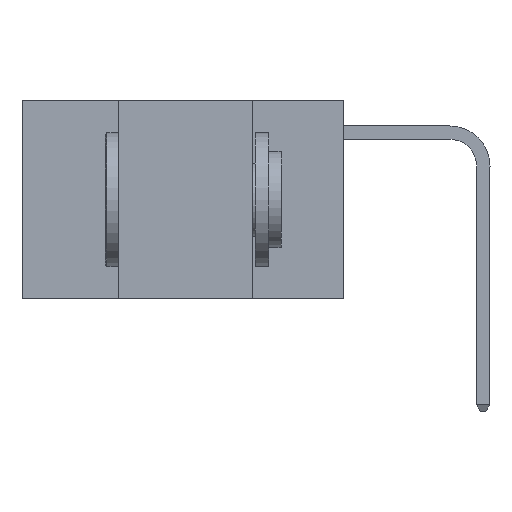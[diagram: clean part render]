
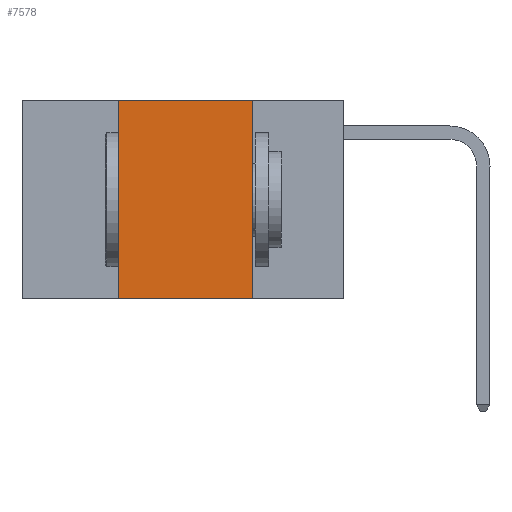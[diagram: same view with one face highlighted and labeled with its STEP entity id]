
A CAD part, left-side view. The second image highlights one B-rep face of the part: STEP entity #7578.
In plain terms, the highlighted planar face has unit normal (-1, 0, 0).
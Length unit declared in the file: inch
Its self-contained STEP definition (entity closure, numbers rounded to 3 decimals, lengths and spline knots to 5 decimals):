
#223 = DIRECTION ( 'NONE',  ( 0., -1., 0. ) ) ;
#427 = CARTESIAN_POINT ( 'NONE',  ( 0., 0.42, 0. ) ) ;
#660 = ORIENTED_EDGE ( 'NONE', *, *, #11744, .T. ) ;
#1587 = CARTESIAN_POINT ( 'NONE',  ( 0., 0.6, -0.37 ) ) ;
#1807 = DIRECTION ( 'NONE',  ( 1., 0., 0. ) ) ;
#2647 = CARTESIAN_POINT ( 'NONE',  ( 0., 0.17, 0. ) ) ;
#3037 = VERTEX_POINT ( 'NONE', #427 ) ;
#3234 = VERTEX_POINT ( 'NONE', #17712 ) ;
#4176 = CARTESIAN_POINT ( 'NONE',  ( 0., 0.17, 0. ) ) ;
#4895 = VECTOR ( 'NONE', #8640, 39.37008 ) ;
#5818 = CARTESIAN_POINT ( 'NONE',  ( 0., 0.42, 0. ) ) ;
#6869 = DIRECTION ( 'NONE',  ( 0., -1., 0. ) ) ;
#7076 = LINE ( 'NONE', #13878, #9054 ) ;
#7261 = EDGE_CURVE ( 'NONE', #3037, #15806, #7076, .T. ) ;
#7578 = ADVANCED_FACE ( 'NONE', ( #12562 ), #10261, .F. ) ;
#7733 = VECTOR ( 'NONE', #11088, 39.37008 ) ;
#7948 = VERTEX_POINT ( 'NONE', #8209 ) ;
#8209 = CARTESIAN_POINT ( 'NONE',  ( 0., 0.42, -0.37 ) ) ;
#8640 = DIRECTION ( 'NONE',  ( 0., 0., 1. ) ) ;
#9052 = LINE ( 'NONE', #2647, #7733 ) ;
#9054 = VECTOR ( 'NONE', #6869, 39.37008 ) ;
#9678 = AXIS2_PLACEMENT_3D ( 'NONE', #15807, #1807, #11671 ) ;
#10261 = PLANE ( 'NONE',  #9678 ) ;
#11088 = DIRECTION ( 'NONE',  ( 0., 0., -1. ) ) ;
#11671 = DIRECTION ( 'NONE',  ( 0., 0., -1. ) ) ;
#11744 = EDGE_CURVE ( 'NONE', #7948, #3234, #17007, .T. ) ;
#11944 = LINE ( 'NONE', #5818, #4895 ) ;
#12147 = ORIENTED_EDGE ( 'NONE', *, *, #7261, .F. ) ;
#12562 = FACE_OUTER_BOUND ( 'NONE', #16855, .T. ) ;
#12680 = EDGE_CURVE ( 'NONE', #7948, #3037, #11944, .T. ) ;
#13269 = ORIENTED_EDGE ( 'NONE', *, *, #13621, .F. ) ;
#13312 = VECTOR ( 'NONE', #223, 39.37008 ) ;
#13621 = EDGE_CURVE ( 'NONE', #15806, #3234, #9052, .T. ) ;
#13878 = CARTESIAN_POINT ( 'NONE',  ( 0., 0.6, 0. ) ) ;
#15806 = VERTEX_POINT ( 'NONE', #4176 ) ;
#15807 = CARTESIAN_POINT ( 'NONE',  ( 0., 0.6, 0. ) ) ;
#16489 = ORIENTED_EDGE ( 'NONE', *, *, #12680, .F. ) ;
#16855 = EDGE_LOOP ( 'NONE', ( #13269, #12147, #16489, #660 ) ) ;
#17007 = LINE ( 'NONE', #1587, #13312 ) ;
#17712 = CARTESIAN_POINT ( 'NONE',  ( 0., 0.17, -0.37 ) ) ;
